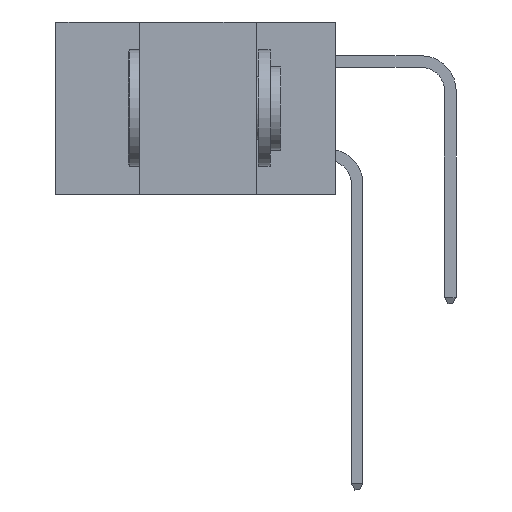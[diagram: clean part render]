
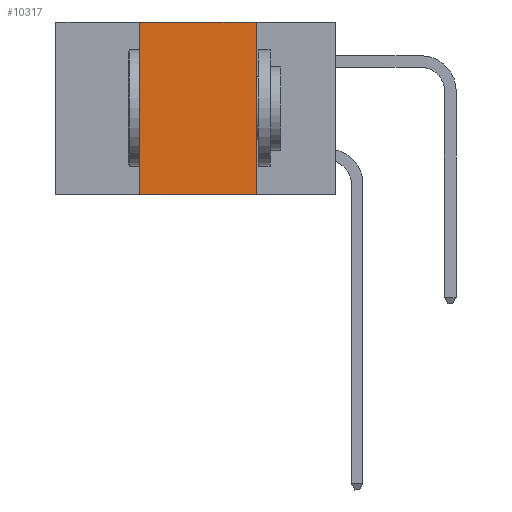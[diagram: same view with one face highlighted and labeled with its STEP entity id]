
A CAD part, left-side view. The second image highlights one B-rep face of the part: STEP entity #10317.
In plain terms, the highlighted planar face has unit normal (-1, 0, 0).
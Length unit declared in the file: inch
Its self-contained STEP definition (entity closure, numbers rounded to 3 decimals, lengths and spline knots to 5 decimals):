
#343 = DIRECTION ( 'NONE',  ( 0., 0., -1. ) ) ;
#824 = ORIENTED_EDGE ( 'NONE', *, *, #23119, .F. ) ;
#901 = LINE ( 'NONE', #11081, #9800 ) ;
#3013 = LINE ( 'NONE', #30304, #6993 ) ;
#3889 = VERTEX_POINT ( 'NONE', #13609 ) ;
#5572 = DIRECTION ( 'NONE',  ( 0., 0., -1. ) ) ;
#6993 = VECTOR ( 'NONE', #36051, 39.37008 ) ;
#7494 = EDGE_CURVE ( 'NONE', #3889, #13177, #3013, .T. ) ;
#9401 = ORIENTED_EDGE ( 'NONE', *, *, #15475, .F. ) ;
#9800 = VECTOR ( 'NONE', #14157, 39.37008 ) ;
#10317 = ADVANCED_FACE ( 'NONE', ( #21127 ), #14250, .F. ) ;
#10546 = VECTOR ( 'NONE', #5572, 39.37008 ) ;
#11081 = CARTESIAN_POINT ( 'NONE',  ( 0., 0.42, 0. ) ) ;
#11155 = LINE ( 'NONE', #16555, #22227 ) ;
#13177 = VERTEX_POINT ( 'NONE', #14284 ) ;
#13530 = VERTEX_POINT ( 'NONE', #31293 ) ;
#13609 = CARTESIAN_POINT ( 'NONE',  ( 0., 0.42, -0.37 ) ) ;
#14132 = DIRECTION ( 'NONE',  ( 0., -1., 0. ) ) ;
#14157 = DIRECTION ( 'NONE',  ( 0., 0., 1. ) ) ;
#14250 = PLANE ( 'NONE',  #18018 ) ;
#14284 = CARTESIAN_POINT ( 'NONE',  ( 0., 0.17, -0.37 ) ) ;
#15475 = EDGE_CURVE ( 'NONE', #3889, #21202, #901, .T. ) ;
#16555 = CARTESIAN_POINT ( 'NONE',  ( 0., 0.6, 0. ) ) ;
#18018 = AXIS2_PLACEMENT_3D ( 'NONE', #19809, #25882, #343 ) ;
#19809 = CARTESIAN_POINT ( 'NONE',  ( 0., 0.6, 0. ) ) ;
#21127 = FACE_OUTER_BOUND ( 'NONE', #22777, .T. ) ;
#21202 = VERTEX_POINT ( 'NONE', #21414 ) ;
#21414 = CARTESIAN_POINT ( 'NONE',  ( 0., 0.42, 0. ) ) ;
#22227 = VECTOR ( 'NONE', #14132, 39.37008 ) ;
#22777 = EDGE_LOOP ( 'NONE', ( #824, #30233, #9401, #31665 ) ) ;
#23119 = EDGE_CURVE ( 'NONE', #13530, #13177, #34051, .T. ) ;
#25102 = EDGE_CURVE ( 'NONE', #21202, #13530, #11155, .T. ) ;
#25882 = DIRECTION ( 'NONE',  ( 1., 0., 0. ) ) ;
#30233 = ORIENTED_EDGE ( 'NONE', *, *, #25102, .F. ) ;
#30304 = CARTESIAN_POINT ( 'NONE',  ( 0., 0.6, -0.37 ) ) ;
#31293 = CARTESIAN_POINT ( 'NONE',  ( 0., 0.17, 0. ) ) ;
#31665 = ORIENTED_EDGE ( 'NONE', *, *, #7494, .T. ) ;
#33948 = CARTESIAN_POINT ( 'NONE',  ( 0., 0.17, 0. ) ) ;
#34051 = LINE ( 'NONE', #33948, #10546 ) ;
#36051 = DIRECTION ( 'NONE',  ( 0., -1., 0. ) ) ;
